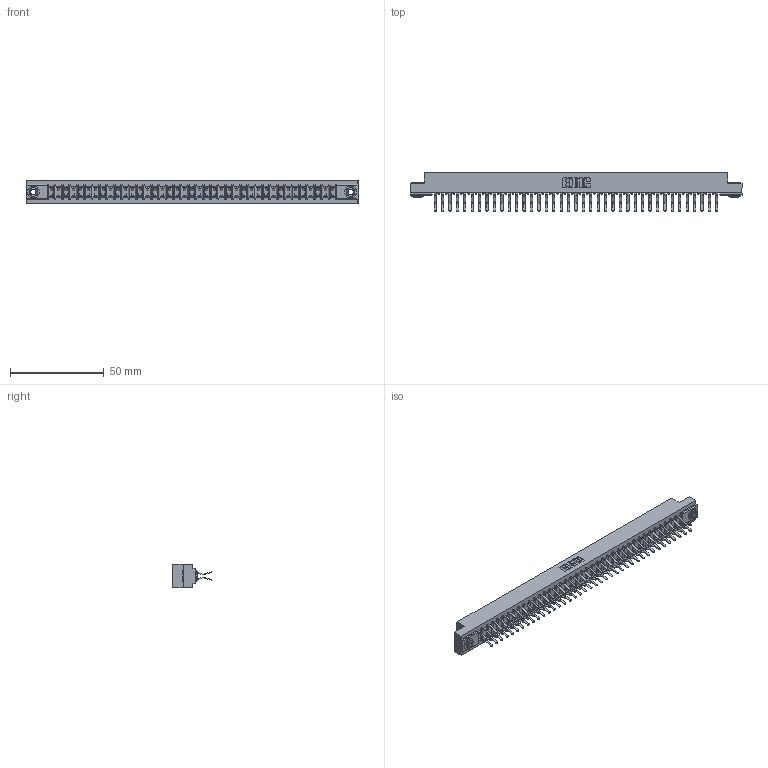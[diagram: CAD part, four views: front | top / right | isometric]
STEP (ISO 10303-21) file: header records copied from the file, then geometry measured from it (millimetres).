
FILE_DESCRIPTION (( 'STEP AP203' ), '1' );
FILE_NAME ('307-078-460-203.STEP', '2020-10-01T07:47:29', ( '' ), ( '' ), 'SwSTEP 2.0', 'SolidWorks 2020', '' );
FILE_SCHEMA (( 'CONFIG_CONTROL_DESIGN' ));
Length unit declared in the file: inch
Products named in the file (4): 307 Part_.156 Dia Mounting Holes; 307-078-460-203; 345-250-002_345-250-002-102; 307-290-001_560
Assembly tree (81 placements, depth 2):
  307-078-460-203
    307 Part_.156 Dia Mounting Holes
    307-290-001_560  x78
    345-250-002_345-250-002-102  x2
Bounding box: 177.55 x 20.73 x 12.7 mm (x, y, z)
Volume: 18957.2 mm3; surface area: 23908.6 mm2
Topology: 81 solids, 81 shells, 4110 faces, 11511 edges, 7458 vertices
Faces by surface type: plane 2668, cylinder 1354, sphere 80, cone 8
Entity records: 36221 total; most frequent: CARTESIAN_POINT 5908, ORIENTED_EDGE 5846, DIRECTION 5803, EDGE_CURVE 2923, VECTOR 2233, LINE 2233, VERTEX_POINT 1890, AXIS2_PLACEMENT_3D 1785
